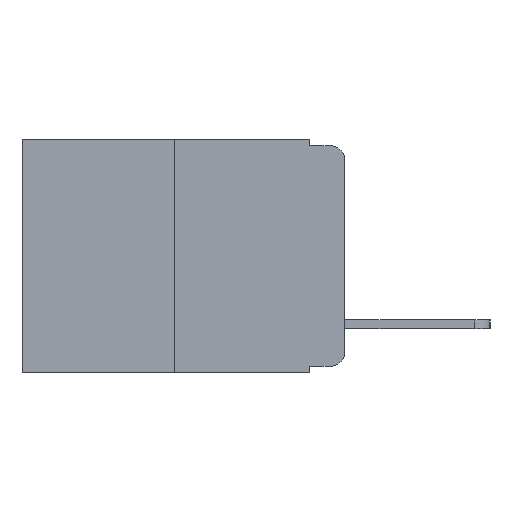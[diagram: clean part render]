
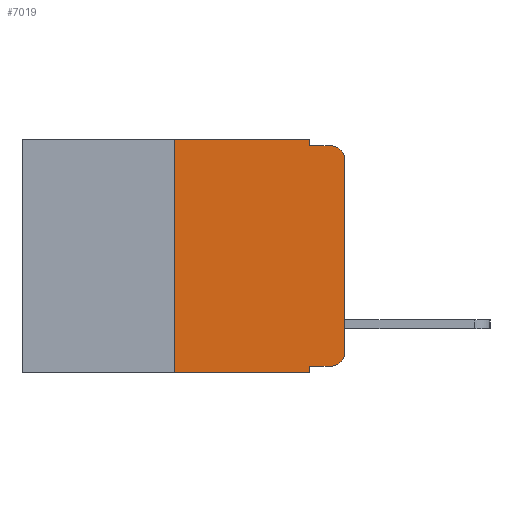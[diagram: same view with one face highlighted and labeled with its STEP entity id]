
A CAD part, left-side view. The second image highlights one B-rep face of the part: STEP entity #7019.
In plain terms, the highlighted planar face has unit normal (-1, 0, 0).
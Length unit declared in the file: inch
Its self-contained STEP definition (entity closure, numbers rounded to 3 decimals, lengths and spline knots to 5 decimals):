
#192 = ORIENTED_EDGE ( 'NONE', *, *, #7531, .F. ) ;
#213 = DIRECTION ( 'NONE',  ( 0., 0., -1. ) ) ;
#236 = EDGE_CURVE ( 'NONE', #10633, #7167, #5487, .T. ) ;
#672 = CARTESIAN_POINT ( 'NONE',  ( 0., 0.051, -0.01 ) ) ;
#705 = ORIENTED_EDGE ( 'NONE', *, *, #10758, .F. ) ;
#727 = LINE ( 'NONE', #7122, #3003 ) ;
#738 = VECTOR ( 'NONE', #9023, 39.37008 ) ;
#1334 = ORIENTED_EDGE ( 'NONE', *, *, #7250, .T. ) ;
#1516 = ORIENTED_EDGE ( 'NONE', *, *, #7307, .F. ) ;
#1548 = VERTEX_POINT ( 'NONE', #3333 ) ;
#1628 = ORIENTED_EDGE ( 'NONE', *, *, #9450, .T. ) ;
#1842 = CIRCLE ( 'NONE', #4563, 0.02 ) ;
#1876 = VERTEX_POINT ( 'NONE', #8822 ) ;
#1925 = VECTOR ( 'NONE', #9354, 39.37008 ) ;
#2212 = CARTESIAN_POINT ( 'NONE',  ( 0., 0.473, 0. ) ) ;
#2229 = ORIENTED_EDGE ( 'NONE', *, *, #6758, .T. ) ;
#2261 = DIRECTION ( 'NONE',  ( 0., -1., 0. ) ) ;
#2436 = CARTESIAN_POINT ( 'NONE',  ( 0., 0.051, 0. ) ) ;
#2450 = DIRECTION ( 'NONE',  ( 0., 0., -1. ) ) ;
#2515 = ORIENTED_EDGE ( 'NONE', *, *, #9468, .T. ) ;
#2908 = LINE ( 'NONE', #3912, #5515 ) ;
#2950 = VERTEX_POINT ( 'NONE', #4373 ) ;
#3003 = VECTOR ( 'NONE', #2261, 39.37008 ) ;
#3207 = DIRECTION ( 'NONE',  ( 1., 0., 0. ) ) ;
#3333 = CARTESIAN_POINT ( 'NONE',  ( 0., 0.25, -0.343 ) ) ;
#3349 = LINE ( 'NONE', #5423, #738 ) ;
#3468 = CIRCLE ( 'NONE', #10322, 0.02 ) ;
#3562 = VERTEX_POINT ( 'NONE', #4475 ) ;
#3787 = DIRECTION ( 'NONE',  ( 0., -1., 0. ) ) ;
#3869 = ORIENTED_EDGE ( 'NONE', *, *, #10078, .T. ) ;
#3912 = CARTESIAN_POINT ( 'NONE',  ( 0., 0.051, 0. ) ) ;
#3929 = DIRECTION ( 'NONE',  ( 0., -1., 0. ) ) ;
#4229 = CARTESIAN_POINT ( 'NONE',  ( 0., 0., 0. ) ) ;
#4373 = CARTESIAN_POINT ( 'NONE',  ( 0., 0.051, -0.333 ) ) ;
#4475 = CARTESIAN_POINT ( 'NONE',  ( 0., 0.051, -0.343 ) ) ;
#4563 = AXIS2_PLACEMENT_3D ( 'NONE', #10632, #5467, #11418 ) ;
#4619 = ORIENTED_EDGE ( 'NONE', *, *, #236, .F. ) ;
#5178 = DIRECTION ( 'NONE',  ( 0., 0., 1. ) ) ;
#5423 = CARTESIAN_POINT ( 'NONE',  ( 0., 0.473, 0. ) ) ;
#5467 = DIRECTION ( 'NONE',  ( -1., 0., 0. ) ) ;
#5487 = LINE ( 'NONE', #2436, #9872 ) ;
#5515 = VECTOR ( 'NONE', #5870, 39.37008 ) ;
#5530 = FACE_OUTER_BOUND ( 'NONE', #11413, .T. ) ;
#5870 = DIRECTION ( 'NONE',  ( 0., 0., -1. ) ) ;
#6077 = CARTESIAN_POINT ( 'NONE',  ( 0., 0.02, -0.333 ) ) ;
#6089 = DIRECTION ( 'NONE',  ( -1., 0., 0. ) ) ;
#6449 = LINE ( 'NONE', #10060, #10638 ) ;
#6624 = VERTEX_POINT ( 'NONE', #6077 ) ;
#6667 = VERTEX_POINT ( 'NONE', #10439 ) ;
#6716 = AXIS2_PLACEMENT_3D ( 'NONE', #2212, #3207, #9601 ) ;
#6758 = EDGE_CURVE ( 'NONE', #6624, #10641, #1842, .T. ) ;
#7019 = ADVANCED_FACE ( 'NONE', ( #5530 ), #7978, .F. ) ;
#7122 = CARTESIAN_POINT ( 'NONE',  ( 0., 0.051, -0.333 ) ) ;
#7167 = VERTEX_POINT ( 'NONE', #672 ) ;
#7250 = EDGE_CURVE ( 'NONE', #1548, #3562, #6449, .T. ) ;
#7307 = EDGE_CURVE ( 'NONE', #2950, #3562, #2908, .T. ) ;
#7531 = EDGE_CURVE ( 'NONE', #7167, #1876, #10861, .T. ) ;
#7723 = CARTESIAN_POINT ( 'NONE',  ( 0., 0.25, 0. ) ) ;
#7788 = ORIENTED_EDGE ( 'NONE', *, *, #8943, .F. ) ;
#7833 = VECTOR ( 'NONE', #5178, 39.37008 ) ;
#7978 = PLANE ( 'NONE',  #6716 ) ;
#8097 = LINE ( 'NONE', #4229, #7833 ) ;
#8776 = VECTOR ( 'NONE', #3929, 39.37008 ) ;
#8822 = CARTESIAN_POINT ( 'NONE',  ( 0., 0.02, -0.01 ) ) ;
#8943 = EDGE_CURVE ( 'NONE', #8989, #10633, #3349, .T. ) ;
#8989 = VERTEX_POINT ( 'NONE', #11451 ) ;
#9023 = DIRECTION ( 'NONE',  ( 0., -1., 0. ) ) ;
#9337 = LINE ( 'NONE', #7723, #1925 ) ;
#9354 = DIRECTION ( 'NONE',  ( 0., 0., 1. ) ) ;
#9450 = EDGE_CURVE ( 'NONE', #2950, #6624, #727, .T. ) ;
#9468 = EDGE_CURVE ( 'NONE', #10641, #6667, #8097, .T. ) ;
#9601 = DIRECTION ( 'NONE',  ( 0., 0., -1. ) ) ;
#9872 = VECTOR ( 'NONE', #2450, 39.37008 ) ;
#10060 = CARTESIAN_POINT ( 'NONE',  ( 0., 0.473, -0.343 ) ) ;
#10078 = EDGE_CURVE ( 'NONE', #6667, #1876, #3468, .T. ) ;
#10176 = CARTESIAN_POINT ( 'NONE',  ( 0., 0.051, -0.01 ) ) ;
#10322 = AXIS2_PLACEMENT_3D ( 'NONE', #11121, #6089, #213 ) ;
#10439 = CARTESIAN_POINT ( 'NONE',  ( 0., 0., -0.03 ) ) ;
#10632 = CARTESIAN_POINT ( 'NONE',  ( 0., 0.02, -0.313 ) ) ;
#10633 = VERTEX_POINT ( 'NONE', #11593 ) ;
#10638 = VECTOR ( 'NONE', #3787, 39.37008 ) ;
#10641 = VERTEX_POINT ( 'NONE', #11561 ) ;
#10758 = EDGE_CURVE ( 'NONE', #1548, #8989, #9337, .T. ) ;
#10861 = LINE ( 'NONE', #10176, #8776 ) ;
#11121 = CARTESIAN_POINT ( 'NONE',  ( 0., 0.02, -0.03 ) ) ;
#11413 = EDGE_LOOP ( 'NONE', ( #2515, #3869, #192, #4619, #7788, #705, #1334, #1516, #1628, #2229 ) ) ;
#11418 = DIRECTION ( 'NONE',  ( 0., 0., -1. ) ) ;
#11451 = CARTESIAN_POINT ( 'NONE',  ( 0., 0.25, 0. ) ) ;
#11561 = CARTESIAN_POINT ( 'NONE',  ( 0., 0., -0.313 ) ) ;
#11593 = CARTESIAN_POINT ( 'NONE',  ( 0., 0.051, 0. ) ) ;
